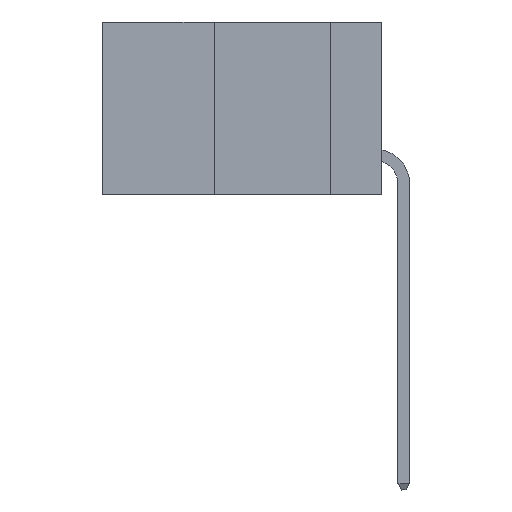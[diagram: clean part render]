
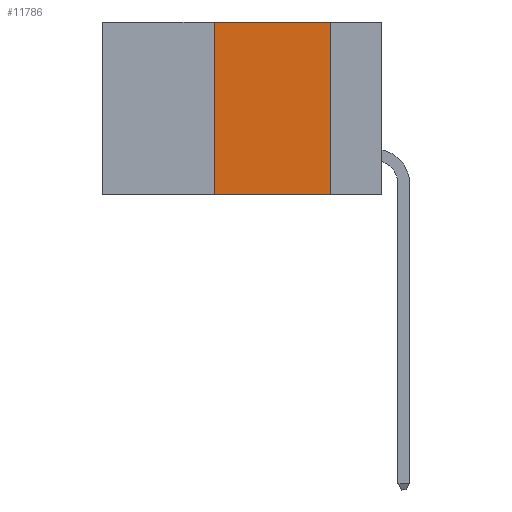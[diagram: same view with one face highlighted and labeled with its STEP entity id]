
A CAD part, left-side view. The second image highlights one B-rep face of the part: STEP entity #11786.
In plain terms, the highlighted planar face has unit normal (-1, 0, 0).
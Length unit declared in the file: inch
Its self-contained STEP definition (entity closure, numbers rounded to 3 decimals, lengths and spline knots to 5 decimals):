
#227 = VECTOR ( 'NONE', #9800, 39.37008 ) ;
#975 = DIRECTION ( 'NONE',  ( 1., 0., 0. ) ) ;
#1245 = EDGE_LOOP ( 'NONE', ( #9544, #2733, #1324, #3123 ) ) ;
#1324 = ORIENTED_EDGE ( 'NONE', *, *, #6452, .F. ) ;
#1373 = VECTOR ( 'NONE', #13407, 39.37008 ) ;
#1463 = CARTESIAN_POINT ( 'NONE',  ( 0., 0.6, 0. ) ) ;
#2184 = PLANE ( 'NONE',  #15152 ) ;
#2733 = ORIENTED_EDGE ( 'NONE', *, *, #9400, .F. ) ;
#3053 = CARTESIAN_POINT ( 'NONE',  ( 0., 0.6, 0. ) ) ;
#3123 = ORIENTED_EDGE ( 'NONE', *, *, #3480, .T. ) ;
#3480 = EDGE_CURVE ( 'NONE', #7743, #13067, #12178, .T. ) ;
#6117 = LINE ( 'NONE', #3053, #227 ) ;
#6452 = EDGE_CURVE ( 'NONE', #7743, #13177, #14452, .T. ) ;
#7743 = VERTEX_POINT ( 'NONE', #12418 ) ;
#8458 = CARTESIAN_POINT ( 'NONE',  ( 0., 0.11, 0. ) ) ;
#8940 = VECTOR ( 'NONE', #14029, 39.37008 ) ;
#9400 = EDGE_CURVE ( 'NONE', #13177, #10005, #6117, .T. ) ;
#9544 = ORIENTED_EDGE ( 'NONE', *, *, #14602, .F. ) ;
#9800 = DIRECTION ( 'NONE',  ( 0., -1., 0. ) ) ;
#10005 = VERTEX_POINT ( 'NONE', #12721 ) ;
#11353 = DIRECTION ( 'NONE',  ( 0., 0., -1. ) ) ;
#11475 = CARTESIAN_POINT ( 'NONE',  ( 0., 0.11, -0.37 ) ) ;
#11786 = ADVANCED_FACE ( 'NONE', ( #16136 ), #2184, .F. ) ;
#12178 = LINE ( 'NONE', #16157, #1373 ) ;
#12418 = CARTESIAN_POINT ( 'NONE',  ( 0., 0.36, -0.37 ) ) ;
#12670 = CARTESIAN_POINT ( 'NONE',  ( 0., 0.36, 0. ) ) ;
#12721 = CARTESIAN_POINT ( 'NONE',  ( 0., 0.11, 0. ) ) ;
#12951 = CARTESIAN_POINT ( 'NONE',  ( 0., 0.36, 0. ) ) ;
#13067 = VERTEX_POINT ( 'NONE', #11475 ) ;
#13177 = VERTEX_POINT ( 'NONE', #12670 ) ;
#13407 = DIRECTION ( 'NONE',  ( 0., -1., 0. ) ) ;
#14029 = DIRECTION ( 'NONE',  ( 0., 0., -1. ) ) ;
#14437 = DIRECTION ( 'NONE',  ( 0., 0., 1. ) ) ;
#14452 = LINE ( 'NONE', #12951, #14902 ) ;
#14602 = EDGE_CURVE ( 'NONE', #10005, #13067, #15165, .T. ) ;
#14902 = VECTOR ( 'NONE', #14437, 39.37008 ) ;
#15152 = AXIS2_PLACEMENT_3D ( 'NONE', #1463, #975, #11353 ) ;
#15165 = LINE ( 'NONE', #8458, #8940 ) ;
#16136 = FACE_OUTER_BOUND ( 'NONE', #1245, .T. ) ;
#16157 = CARTESIAN_POINT ( 'NONE',  ( 0., 0.6, -0.37 ) ) ;
